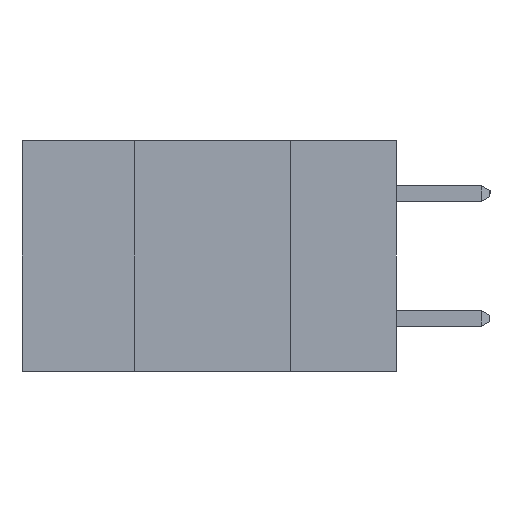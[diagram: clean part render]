
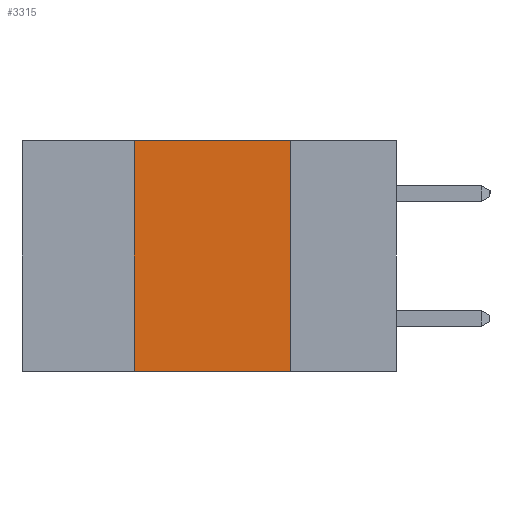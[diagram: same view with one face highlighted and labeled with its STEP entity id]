
A CAD part, left-side view. The second image highlights one B-rep face of the part: STEP entity #3315.
In plain terms, the highlighted planar face has unit normal (-1, 0, 0).
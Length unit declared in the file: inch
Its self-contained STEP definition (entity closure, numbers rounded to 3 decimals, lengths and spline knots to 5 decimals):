
#728 = DIRECTION ( 'NONE',  ( 0., -1., 0. ) ) ;
#829 = EDGE_CURVE ( 'NONE', #18111, #5047, #18503, .T. ) ;
#1383 = DIRECTION ( 'NONE',  ( 0., -1., 0. ) ) ;
#2129 = VECTOR ( 'NONE', #15430, 39.37008 ) ;
#2302 = ORIENTED_EDGE ( 'NONE', *, *, #15361, .F. ) ;
#3159 = AXIS2_PLACEMENT_3D ( 'NONE', #5038, #17551, #20690 ) ;
#3315 = ADVANCED_FACE ( 'NONE', ( #13562 ), #10070, .F. ) ;
#3627 = DIRECTION ( 'NONE',  ( 0., 0., 1. ) ) ;
#5038 = CARTESIAN_POINT ( 'NONE',  ( 0., 0.6, 0. ) ) ;
#5047 = VERTEX_POINT ( 'NONE', #13194 ) ;
#5609 = CARTESIAN_POINT ( 'NONE',  ( 0., 0.42, 0. ) ) ;
#6074 = VECTOR ( 'NONE', #3627, 39.37008 ) ;
#6460 = LINE ( 'NONE', #14971, #2129 ) ;
#6666 = CARTESIAN_POINT ( 'NONE',  ( 0., 0.6, 0. ) ) ;
#7434 = VECTOR ( 'NONE', #728, 39.37008 ) ;
#8112 = VERTEX_POINT ( 'NONE', #5609 ) ;
#8117 = ORIENTED_EDGE ( 'NONE', *, *, #12284, .F. ) ;
#9541 = CARTESIAN_POINT ( 'NONE',  ( 0., 0.42, -0.37 ) ) ;
#10070 = PLANE ( 'NONE',  #3159 ) ;
#10296 = ORIENTED_EDGE ( 'NONE', *, *, #21711, .F. ) ;
#11199 = CARTESIAN_POINT ( 'NONE',  ( 0., 0.42, -0.37 ) ) ;
#11472 = VERTEX_POINT ( 'NONE', #20878 ) ;
#11907 = LINE ( 'NONE', #6666, #14901 ) ;
#12284 = EDGE_CURVE ( 'NONE', #11472, #5047, #6460, .T. ) ;
#13194 = CARTESIAN_POINT ( 'NONE',  ( 0., 0.17, -0.37 ) ) ;
#13562 = FACE_OUTER_BOUND ( 'NONE', #22098, .T. ) ;
#13856 = ORIENTED_EDGE ( 'NONE', *, *, #829, .T. ) ;
#14794 = LINE ( 'NONE', #9541, #6074 ) ;
#14901 = VECTOR ( 'NONE', #1383, 39.37008 ) ;
#14971 = CARTESIAN_POINT ( 'NONE',  ( 0., 0.17, -0.37 ) ) ;
#15361 = EDGE_CURVE ( 'NONE', #8112, #11472, #11907, .T. ) ;
#15430 = DIRECTION ( 'NONE',  ( 0., 0., -1. ) ) ;
#17551 = DIRECTION ( 'NONE',  ( 1., 0., 0. ) ) ;
#18111 = VERTEX_POINT ( 'NONE', #11199 ) ;
#18503 = LINE ( 'NONE', #18731, #7434 ) ;
#18731 = CARTESIAN_POINT ( 'NONE',  ( 0., 0.6, -0.37 ) ) ;
#20690 = DIRECTION ( 'NONE',  ( 0., 0., -1. ) ) ;
#20878 = CARTESIAN_POINT ( 'NONE',  ( 0., 0.17, 0. ) ) ;
#21711 = EDGE_CURVE ( 'NONE', #18111, #8112, #14794, .T. ) ;
#22098 = EDGE_LOOP ( 'NONE', ( #8117, #2302, #10296, #13856 ) ) ;
